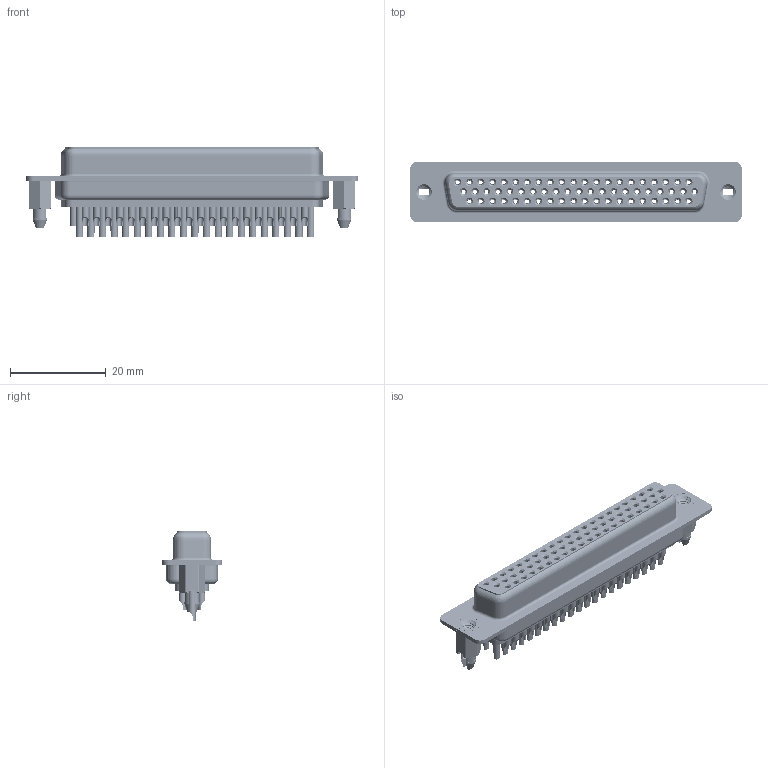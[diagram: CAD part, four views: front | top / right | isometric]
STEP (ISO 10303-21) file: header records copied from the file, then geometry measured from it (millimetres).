
FILE_DESCRIPTION (( 'STEP AP203' ), '1' );
FILE_NAME ('638-062-232-246.STEP', '2020-07-19T01:25:37', ( '' ), ( '' ), 'SwSTEP 2.0', 'SolidWorks 2020', '' );
FILE_SCHEMA (( 'CONFIG_CONTROL_DESIGN' ));
Length unit declared in the file: millimetre
Products named in the file (8): 638 Contact Row 2_32; 638 Shell Rear_62 Contacts; 638 Contact Row 1_32; 638 4-40 Threaded Boardlock_LP; 638 Shell Front_62 Contacts; 638 Housing_62 Contacts; 638-062-232-246; 638 Contact Row 3_32
Assembly tree (67 placements, depth 2):
  638-062-232-246
    638 Housing_62 Contacts
    638 Shell Front_62 Contacts
    638 Shell Rear_62 Contacts
    638 Contact Row 1_32  x21
    638 Contact Row 2_32  x21
    638 Contact Row 3_32  x20
    638 4-40 Threaded Boardlock_LP  x2
Bounding box: 69.32 x 12.6 x 18.6 mm (x, y, z)
Volume: 4823 mm3; surface area: 18839.2 mm2
Topology: 67 solids, 67 shells, 5871 faces, 14929 edges, 9387 vertices
Faces by surface type: cylinder 1719, plane 1401, bspline 1246, torus 1173, cone 332
Entity records: 44276 total; most frequent: CARTESIAN_POINT 10814, DIRECTION 6962, ORIENTED_EDGE 6100, EDGE_CURVE 3050, AXIS2_PLACEMENT_3D 2939, VERTEX_POINT 1941, EDGE_LOOP 1649, CIRCLE 1615
